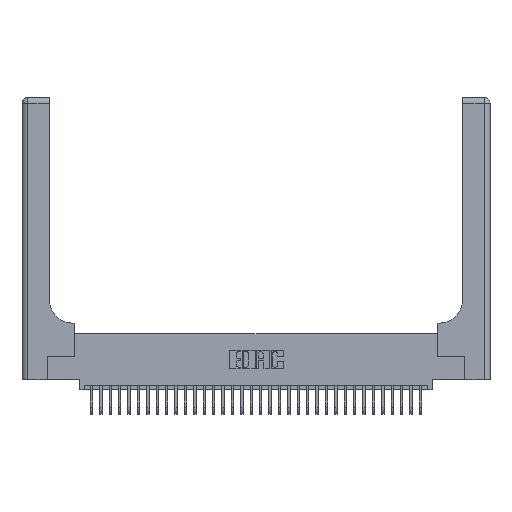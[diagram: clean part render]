
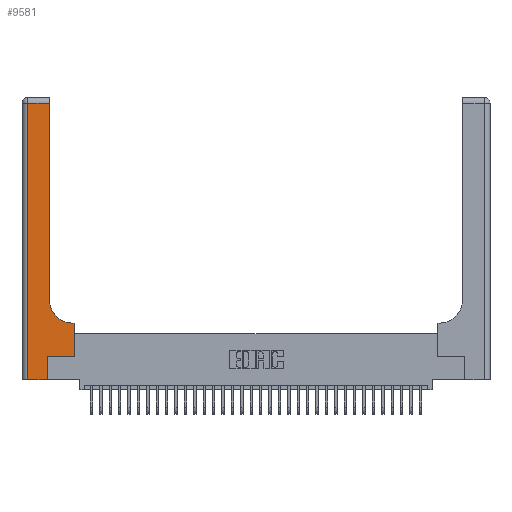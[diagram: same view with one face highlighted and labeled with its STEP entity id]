
A CAD part, top view. The second image highlights one B-rep face of the part: STEP entity #9581.
In plain terms, the highlighted planar face has unit normal (0, 0, 1).
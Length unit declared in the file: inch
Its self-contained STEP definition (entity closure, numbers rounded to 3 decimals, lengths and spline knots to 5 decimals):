
#215 = VERTEX_POINT ( 'NONE', #13835 ) ;
#306 = CARTESIAN_POINT ( 'NONE',  ( 0.5415, 0.85, 0.37 ) ) ;
#421 = VERTEX_POINT ( 'NONE', #28382 ) ;
#777 = VECTOR ( 'NONE', #9020, 39.37008 ) ;
#1208 = VECTOR ( 'NONE', #8882, 39.37008 ) ;
#1868 = LINE ( 'NONE', #8370, #3670 ) ;
#2941 = ORIENTED_EDGE ( 'NONE', *, *, #9541, .T. ) ;
#3162 = EDGE_CURVE ( 'NONE', #421, #215, #16164, .T. ) ;
#3206 = DIRECTION ( 'NONE',  ( 1., 0., 0. ) ) ;
#3326 = CARTESIAN_POINT ( 'NONE',  ( 0.5585, 0.25, 0.37 ) ) ;
#3398 = ORIENTED_EDGE ( 'NONE', *, *, #6509, .T. ) ;
#3622 = CARTESIAN_POINT ( 'NONE',  ( 0.2915, 3., 0.37 ) ) ;
#3670 = VECTOR ( 'NONE', #27807, 39.37008 ) ;
#4059 = AXIS2_PLACEMENT_3D ( 'NONE', #306, #19982, #3206 ) ;
#4203 = VERTEX_POINT ( 'NONE', #24316 ) ;
#5886 = AXIS2_PLACEMENT_3D ( 'NONE', #6342, #9144, #28574 ) ;
#6342 = CARTESIAN_POINT ( 'NONE',  ( 0., 3., 0.37 ) ) ;
#6509 = EDGE_CURVE ( 'NONE', #30186, #32408, #15549, .T. ) ;
#7037 = VECTOR ( 'NONE', #25940, 39.37008 ) ;
#7520 = EDGE_CURVE ( 'NONE', #16785, #421, #28503, .T. ) ;
#8260 = ORIENTED_EDGE ( 'NONE', *, *, #3162, .T. ) ;
#8267 = LINE ( 'NONE', #3326, #35940 ) ;
#8350 = LINE ( 'NONE', #25719, #777 ) ;
#8370 = CARTESIAN_POINT ( 'NONE',  ( 0., 2.94, 0.37 ) ) ;
#8658 = ORIENTED_EDGE ( 'NONE', *, *, #30208, .T. ) ;
#8882 = DIRECTION ( 'NONE',  ( 1., 0., 0. ) ) ;
#9020 = DIRECTION ( 'NONE',  ( 0., -1., 0. ) ) ;
#9144 = DIRECTION ( 'NONE',  ( 0., 0., -1. ) ) ;
#9541 = EDGE_CURVE ( 'NONE', #15877, #4203, #8350, .T. ) ;
#9581 = ADVANCED_FACE ( 'NONE', ( #13998 ), #33966, .F. ) ;
#9769 = CARTESIAN_POINT ( 'NONE',  ( 0.269, 0., 0.37 ) ) ;
#11402 = LINE ( 'NONE', #35652, #20578 ) ;
#12970 = CARTESIAN_POINT ( 'NONE',  ( 0.06, 2.94, 0.37 ) ) ;
#13026 = ORIENTED_EDGE ( 'NONE', *, *, #33944, .T. ) ;
#13835 = CARTESIAN_POINT ( 'NONE',  ( 0.5585, 0.25, 0.37 ) ) ;
#13998 = FACE_OUTER_BOUND ( 'NONE', #18471, .T. ) ;
#15549 = CIRCLE ( 'NONE', #4059, 0.25 ) ;
#15643 = ORIENTED_EDGE ( 'NONE', *, *, #27840, .T. ) ;
#15877 = VERTEX_POINT ( 'NONE', #12970 ) ;
#16164 = LINE ( 'NONE', #25578, #1208 ) ;
#16785 = VERTEX_POINT ( 'NONE', #28276 ) ;
#17421 = ORIENTED_EDGE ( 'NONE', *, *, #35551, .T. ) ;
#18471 = EDGE_LOOP ( 'NONE', ( #29901, #8658, #2941, #13026, #27821, #8260, #15643, #17421, #3398 ) ) ;
#19211 = DIRECTION ( 'NONE',  ( -1., 0., 0. ) ) ;
#19363 = CARTESIAN_POINT ( 'NONE',  ( 0.5415, 0.6, 0.37 ) ) ;
#19982 = DIRECTION ( 'NONE',  ( 0., 0., -1. ) ) ;
#20298 = VECTOR ( 'NONE', #34801, 39.37008 ) ;
#20578 = VECTOR ( 'NONE', #19211, 39.37008 ) ;
#21683 = EDGE_CURVE ( 'NONE', #32408, #30447, #21956, .T. ) ;
#21956 = LINE ( 'NONE', #3622, #7037 ) ;
#22047 = CARTESIAN_POINT ( 'NONE',  ( 0.2915, 0.85, 0.37 ) ) ;
#22300 = VECTOR ( 'NONE', #34441, 39.37008 ) ;
#23459 = CARTESIAN_POINT ( 'NONE',  ( 0., 0., 0.37 ) ) ;
#24316 = CARTESIAN_POINT ( 'NONE',  ( 0.06, 0., 0.37 ) ) ;
#25409 = VERTEX_POINT ( 'NONE', #27398 ) ;
#25578 = CARTESIAN_POINT ( 'NONE',  ( 0.269, 0.25, 0.37 ) ) ;
#25676 = DIRECTION ( 'NONE',  ( 0., 1., 0. ) ) ;
#25719 = CARTESIAN_POINT ( 'NONE',  ( 0.06, 3., 0.37 ) ) ;
#25940 = DIRECTION ( 'NONE',  ( 0., 1., 0. ) ) ;
#27398 = CARTESIAN_POINT ( 'NONE',  ( 0.5585, 0.6, 0.37 ) ) ;
#27807 = DIRECTION ( 'NONE',  ( -1., 0., 0. ) ) ;
#27821 = ORIENTED_EDGE ( 'NONE', *, *, #7520, .T. ) ;
#27840 = EDGE_CURVE ( 'NONE', #215, #25409, #8267, .T. ) ;
#28276 = CARTESIAN_POINT ( 'NONE',  ( 0.269, 0., 0.37 ) ) ;
#28382 = CARTESIAN_POINT ( 'NONE',  ( 0.269, 0.25, 0.37 ) ) ;
#28503 = LINE ( 'NONE', #9769, #20298 ) ;
#28574 = DIRECTION ( 'NONE',  ( -1., 0., 0. ) ) ;
#29533 = LINE ( 'NONE', #23459, #22300 ) ;
#29901 = ORIENTED_EDGE ( 'NONE', *, *, #21683, .T. ) ;
#30186 = VERTEX_POINT ( 'NONE', #19363 ) ;
#30208 = EDGE_CURVE ( 'NONE', #30447, #15877, #1868, .T. ) ;
#30447 = VERTEX_POINT ( 'NONE', #32651 ) ;
#32408 = VERTEX_POINT ( 'NONE', #22047 ) ;
#32651 = CARTESIAN_POINT ( 'NONE',  ( 0.2915, 2.94, 0.37 ) ) ;
#33944 = EDGE_CURVE ( 'NONE', #4203, #16785, #29533, .T. ) ;
#33966 = PLANE ( 'NONE',  #5886 ) ;
#34441 = DIRECTION ( 'NONE',  ( 1., 0., 0. ) ) ;
#34801 = DIRECTION ( 'NONE',  ( 0., 1., 0. ) ) ;
#35551 = EDGE_CURVE ( 'NONE', #25409, #30186, #11402, .T. ) ;
#35652 = CARTESIAN_POINT ( 'NONE',  ( 0.2915, 0.6, 0.37 ) ) ;
#35940 = VECTOR ( 'NONE', #25676, 39.37008 ) ;
